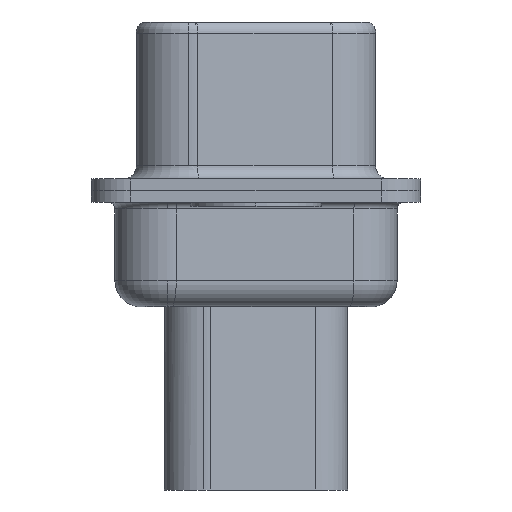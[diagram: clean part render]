
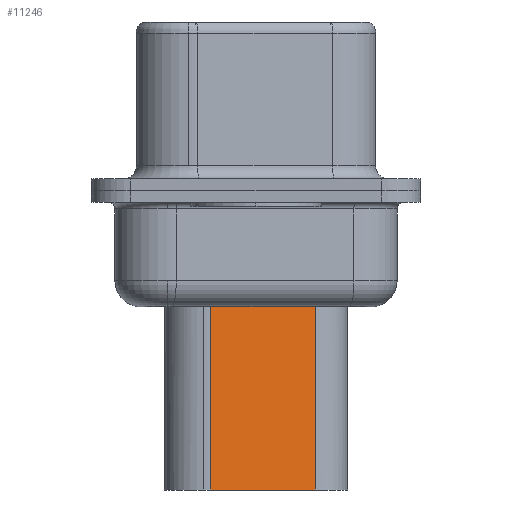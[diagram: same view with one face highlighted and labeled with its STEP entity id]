
A CAD part, left-side view. The second image highlights one B-rep face of the part: STEP entity #11246.
In plain terms, the highlighted planar face has unit normal (-0.985, -0.174, 0).
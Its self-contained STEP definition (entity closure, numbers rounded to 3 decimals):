
#300 = CARTESIAN_POINT ( 'NONE',  ( 5.229, -2.26, -11.45 ) ) ;
#367 = VECTOR ( 'NONE', #9994, 1000. ) ;
#805 = LINE ( 'NONE', #10628, #16473 ) ;
#857 = LINE ( 'NONE', #10060, #367 ) ;
#1384 = AXIS2_PLACEMENT_3D ( 'NONE', #1455, #7809, #18780 ) ;
#1455 = CARTESIAN_POINT ( 'NONE',  ( 4.524, 1.74, -3.1 ) ) ;
#1662 = DIRECTION ( 'NONE',  ( 0., 0., -1. ) ) ;
#1725 = EDGE_CURVE ( 'NONE', #2816, #2492, #18090, .T. ) ;
#2492 = VERTEX_POINT ( 'NONE', #10848 ) ;
#2589 = LINE ( 'NONE', #6639, #6250 ) ;
#2731 = ORIENTED_EDGE ( 'NONE', *, *, #4756, .F. ) ;
#2816 = VERTEX_POINT ( 'NONE', #300 ) ;
#4504 = CARTESIAN_POINT ( 'NONE',  ( 4.524, 1.74, -3.975 ) ) ;
#4756 = EDGE_CURVE ( 'NONE', #19185, #2816, #2589, .T. ) ;
#5130 = CARTESIAN_POINT ( 'NONE',  ( 5.229, -2.26, -3.975 ) ) ;
#6224 = PLANE ( 'NONE',  #1384 ) ;
#6250 = VECTOR ( 'NONE', #1662, 1000. ) ;
#6639 = CARTESIAN_POINT ( 'NONE',  ( 5.229, -2.26, -3.1 ) ) ;
#7390 = ORIENTED_EDGE ( 'NONE', *, *, #1725, .F. ) ;
#7809 = DIRECTION ( 'NONE',  ( -0.985, -0.174, 0. ) ) ;
#8660 = VERTEX_POINT ( 'NONE', #4504 ) ;
#9994 = DIRECTION ( 'NONE',  ( -0.174, 0.985, 0. ) ) ;
#10060 = CARTESIAN_POINT ( 'NONE',  ( 4.353, 2.709, -3.975 ) ) ;
#10628 = CARTESIAN_POINT ( 'NONE',  ( 4.524, 1.74, -3.1 ) ) ;
#10848 = CARTESIAN_POINT ( 'NONE',  ( 4.524, 1.74, -11.45 ) ) ;
#11246 = ADVANCED_FACE ( 'NONE', ( #11404 ), #6224, .T. ) ;
#11404 = FACE_OUTER_BOUND ( 'NONE', #19333, .T. ) ;
#11851 = ORIENTED_EDGE ( 'NONE', *, *, #15911, .T. ) ;
#12222 = DIRECTION ( 'NONE',  ( 0., 0., -1. ) ) ;
#13941 = VECTOR ( 'NONE', #14265, 1000. ) ;
#14265 = DIRECTION ( 'NONE',  ( -0.174, 0.985, 0. ) ) ;
#15911 = EDGE_CURVE ( 'NONE', #8660, #2492, #805, .T. ) ;
#16473 = VECTOR ( 'NONE', #12222, 1000. ) ;
#17228 = CARTESIAN_POINT ( 'NONE',  ( 4.524, 1.74, -11.45 ) ) ;
#18090 = LINE ( 'NONE', #17228, #13941 ) ;
#18467 = ORIENTED_EDGE ( 'NONE', *, *, #18670, .T. ) ;
#18670 = EDGE_CURVE ( 'NONE', #19185, #8660, #857, .T. ) ;
#18780 = DIRECTION ( 'NONE',  ( 0.174, -0.985, 0. ) ) ;
#19185 = VERTEX_POINT ( 'NONE', #5130 ) ;
#19333 = EDGE_LOOP ( 'NONE', ( #2731, #18467, #11851, #7390 ) ) ;
